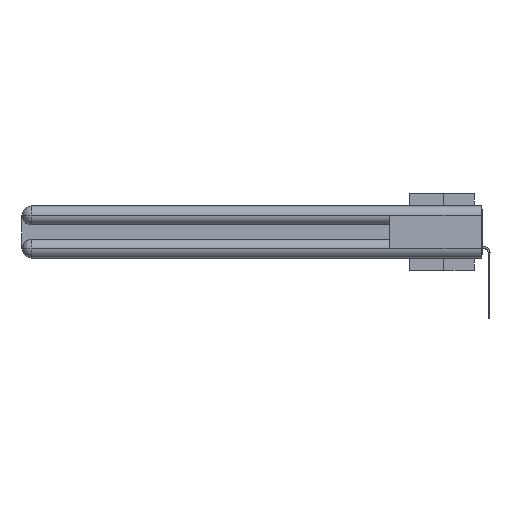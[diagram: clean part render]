
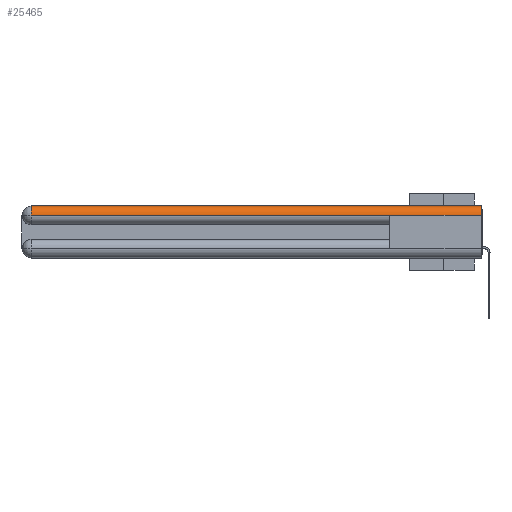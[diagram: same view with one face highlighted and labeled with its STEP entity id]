
A CAD part, left-side view. The second image highlights one B-rep face of the part: STEP entity #25465.
In plain terms, the highlighted cylindrical face has radius 1.562 mm (diameter 3.124 mm), a partial arc.
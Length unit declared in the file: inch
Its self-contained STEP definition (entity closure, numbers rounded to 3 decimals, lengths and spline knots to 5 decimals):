
#19 = CARTESIAN_POINT ( 'NONE',  ( 0.0615, 0., 0. ) ) ;
#196 = ORIENTED_EDGE ( 'NONE', *, *, #28756, .T. ) ;
#1078 = CARTESIAN_POINT ( 'NONE',  ( 0., 2.94, -0.0615 ) ) ;
#2918 = EDGE_CURVE ( 'NONE', #11849, #3362, #23523, .T. ) ;
#3362 = VERTEX_POINT ( 'NONE', #1078 ) ;
#5109 = CARTESIAN_POINT ( 'NONE',  ( 0.0615, 0., -0.0615 ) ) ;
#5432 = CARTESIAN_POINT ( 'NONE',  ( 0., 3., -0.0615 ) ) ;
#5679 = DIRECTION ( 'NONE',  ( 0., 0., 1. ) ) ;
#6812 = AXIS2_PLACEMENT_3D ( 'NONE', #21661, #18986, #5679 ) ;
#6854 = CARTESIAN_POINT ( 'NONE',  ( 0.0615, 2.94, 0. ) ) ;
#7960 = CARTESIAN_POINT ( 'NONE',  ( 0., 0.6, -0.0615 ) ) ;
#8204 = AXIS2_PLACEMENT_3D ( 'NONE', #19775, #22615, #8585 ) ;
#8585 = DIRECTION ( 'NONE',  ( 0., 0., 1. ) ) ;
#10810 = CYLINDRICAL_SURFACE ( 'NONE', #6812, 0.0615 ) ;
#10909 = LINE ( 'NONE', #5432, #25798 ) ;
#11849 = VERTEX_POINT ( 'NONE', #6854 ) ;
#12166 = LINE ( 'NONE', #25362, #22568 ) ;
#12446 = VERTEX_POINT ( 'NONE', #19 ) ;
#12808 = CARTESIAN_POINT ( 'NONE',  ( 0.0615, 0., 0. ) ) ;
#13254 = EDGE_CURVE ( 'NONE', #29805, #23708, #10909, .T. ) ;
#15312 = DIRECTION ( 'NONE',  ( 0., -1., 0. ) ) ;
#15492 = ORIENTED_EDGE ( 'NONE', *, *, #30225, .F. ) ;
#16249 = DIRECTION ( 'NONE',  ( 0., 1., 0. ) ) ;
#16704 = VECTOR ( 'NONE', #15312, 39.37008 ) ;
#16915 = ORIENTED_EDGE ( 'NONE', *, *, #13254, .F. ) ;
#16983 = EDGE_LOOP ( 'NONE', ( #31884, #22126, #196, #16915, #15492 ) ) ;
#17163 = AXIS2_PLACEMENT_3D ( 'NONE', #5109, #26774, #34737 ) ;
#18986 = DIRECTION ( 'NONE',  ( 0., 1., 0. ) ) ;
#19775 = CARTESIAN_POINT ( 'NONE',  ( 0.0615, 2.94, -0.0615 ) ) ;
#20366 = DIRECTION ( 'NONE',  ( 0., -1., 0. ) ) ;
#21661 = CARTESIAN_POINT ( 'NONE',  ( 0.0615, 0., -0.0615 ) ) ;
#22126 = ORIENTED_EDGE ( 'NONE', *, *, #2918, .T. ) ;
#22568 = VECTOR ( 'NONE', #20366, 39.37008 ) ;
#22615 = DIRECTION ( 'NONE',  ( 0., -1., 0. ) ) ;
#23523 = CIRCLE ( 'NONE', #8204, 0.0615 ) ;
#23708 = VERTEX_POINT ( 'NONE', #7960 ) ;
#25362 = CARTESIAN_POINT ( 'NONE',  ( 0., 3., -0.0615 ) ) ;
#25465 = ADVANCED_FACE ( 'NONE', ( #30029 ), #10810, .T. ) ;
#25798 = VECTOR ( 'NONE', #16249, 39.37008 ) ;
#26774 = DIRECTION ( 'NONE',  ( 0., -1., 0. ) ) ;
#27324 = CARTESIAN_POINT ( 'NONE',  ( 0., 0., -0.0615 ) ) ;
#28756 = EDGE_CURVE ( 'NONE', #3362, #23708, #12166, .T. ) ;
#29805 = VERTEX_POINT ( 'NONE', #27324 ) ;
#30029 = FACE_OUTER_BOUND ( 'NONE', #16983, .T. ) ;
#30225 = EDGE_CURVE ( 'NONE', #12446, #29805, #30259, .T. ) ;
#30259 = CIRCLE ( 'NONE', #17163, 0.0615 ) ;
#31884 = ORIENTED_EDGE ( 'NONE', *, *, #32597, .F. ) ;
#32391 = LINE ( 'NONE', #12808, #16704 ) ;
#32597 = EDGE_CURVE ( 'NONE', #11849, #12446, #32391, .T. ) ;
#34737 = DIRECTION ( 'NONE',  ( 1., 0., 0. ) ) ;
